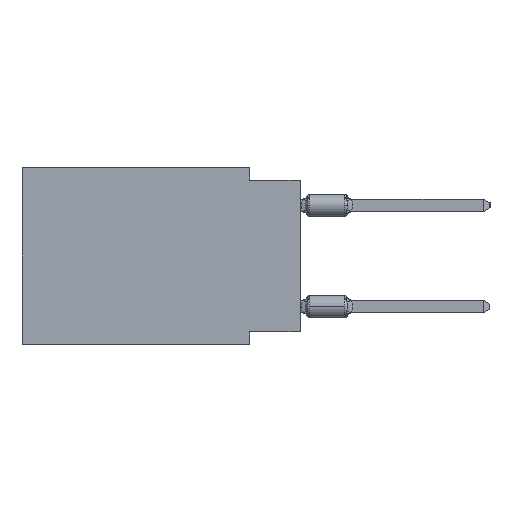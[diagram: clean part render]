
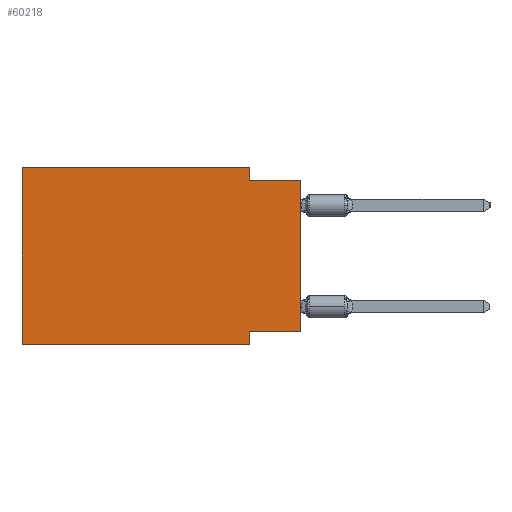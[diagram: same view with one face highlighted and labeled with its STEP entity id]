
A CAD part, left-side view. The second image highlights one B-rep face of the part: STEP entity #60218.
In plain terms, the highlighted planar face has unit normal (-1, 0, 0).
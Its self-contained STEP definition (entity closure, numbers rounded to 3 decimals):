
#1764 = CARTESIAN_POINT ( 'NONE',  ( 0., 0., -0.635 ) ) ;
#2218 = ORIENTED_EDGE ( 'NONE', *, *, #30671, .F. ) ;
#2288 = CARTESIAN_POINT ( 'NONE',  ( 0., 2.54, -8.89 ) ) ;
#2795 = ORIENTED_EDGE ( 'NONE', *, *, #37087, .T. ) ;
#5385 = DIRECTION ( 'NONE',  ( 0., 1., 0. ) ) ;
#5557 = VECTOR ( 'NONE', #57499, 1000. ) ;
#5923 = CARTESIAN_POINT ( 'NONE',  ( 0., 13.97, 0. ) ) ;
#6159 = CARTESIAN_POINT ( 'NONE',  ( 0., 13.97, -8.89 ) ) ;
#7140 = VERTEX_POINT ( 'NONE', #58990 ) ;
#9269 = PLANE ( 'NONE',  #31322 ) ;
#9578 = DIRECTION ( 'NONE',  ( 1., 0., 0. ) ) ;
#13674 = EDGE_CURVE ( 'NONE', #46646, #24754, #45529, .T. ) ;
#14096 = CARTESIAN_POINT ( 'NONE',  ( 0., 2.54, -8.89 ) ) ;
#14541 = ORIENTED_EDGE ( 'NONE', *, *, #25486, .T. ) ;
#15211 = ORIENTED_EDGE ( 'NONE', *, *, #61394, .F. ) ;
#15322 = VERTEX_POINT ( 'NONE', #14096 ) ;
#15597 = ORIENTED_EDGE ( 'NONE', *, *, #13674, .F. ) ;
#15773 = DIRECTION ( 'NONE',  ( 0., 0., 1. ) ) ;
#16227 = CARTESIAN_POINT ( 'NONE',  ( 0., 0., -8.255 ) ) ;
#18901 = CARTESIAN_POINT ( 'NONE',  ( 0., 13.97, 0. ) ) ;
#20080 = CARTESIAN_POINT ( 'NONE',  ( 0., 13.97, 0. ) ) ;
#21241 = DIRECTION ( 'NONE',  ( 0., 0., -1. ) ) ;
#22351 = CARTESIAN_POINT ( 'NONE',  ( 0., 0., -0.635 ) ) ;
#24740 = ORIENTED_EDGE ( 'NONE', *, *, #30100, .F. ) ;
#24754 = VERTEX_POINT ( 'NONE', #41744 ) ;
#24932 = ORIENTED_EDGE ( 'NONE', *, *, #27989, .F. ) ;
#25095 = VERTEX_POINT ( 'NONE', #38627 ) ;
#25486 = EDGE_CURVE ( 'NONE', #7140, #15322, #48722, .T. ) ;
#27989 = EDGE_CURVE ( 'NONE', #52520, #46646, #52221, .T. ) ;
#29491 = ORIENTED_EDGE ( 'NONE', *, *, #39081, .F. ) ;
#29633 = LINE ( 'NONE', #2288, #57215 ) ;
#30100 = EDGE_CURVE ( 'NONE', #7140, #52520, #43373, .T. ) ;
#30504 = VECTOR ( 'NONE', #34737, 1000. ) ;
#30671 = EDGE_CURVE ( 'NONE', #25095, #15322, #29633, .T. ) ;
#31322 = AXIS2_PLACEMENT_3D ( 'NONE', #18901, #9578, #40415 ) ;
#34737 = DIRECTION ( 'NONE',  ( 0., -1., 0. ) ) ;
#36470 = VECTOR ( 'NONE', #15773, 1000. ) ;
#36815 = DIRECTION ( 'NONE',  ( 0., 0., -1. ) ) ;
#37087 = EDGE_CURVE ( 'NONE', #42439, #51017, #59231, .T. ) ;
#38627 = CARTESIAN_POINT ( 'NONE',  ( 0., 2.54, -8.255 ) ) ;
#38903 = CARTESIAN_POINT ( 'NONE',  ( 0., 2.54, 0. ) ) ;
#39081 = EDGE_CURVE ( 'NONE', #42439, #25095, #42354, .T. ) ;
#39440 = VECTOR ( 'NONE', #48341, 1000. ) ;
#40415 = DIRECTION ( 'NONE',  ( 0., 0., -1. ) ) ;
#41550 = CARTESIAN_POINT ( 'NONE',  ( 0., 13.97, 0. ) ) ;
#41744 = CARTESIAN_POINT ( 'NONE',  ( 0., 2.54, -0.635 ) ) ;
#42354 = LINE ( 'NONE', #56957, #54360 ) ;
#42439 = VERTEX_POINT ( 'NONE', #16227 ) ;
#43373 = LINE ( 'NONE', #20080, #39440 ) ;
#44039 = CARTESIAN_POINT ( 'NONE',  ( 0., 0., 0. ) ) ;
#44750 = LINE ( 'NONE', #22351, #48274 ) ;
#45529 = LINE ( 'NONE', #60423, #47590 ) ;
#46646 = VERTEX_POINT ( 'NONE', #38903 ) ;
#46859 = FACE_OUTER_BOUND ( 'NONE', #58295, .T. ) ;
#47590 = VECTOR ( 'NONE', #36815, 1000. ) ;
#48274 = VECTOR ( 'NONE', #49401, 1000. ) ;
#48341 = DIRECTION ( 'NONE',  ( 0., 0., 1. ) ) ;
#48722 = LINE ( 'NONE', #6159, #30504 ) ;
#49401 = DIRECTION ( 'NONE',  ( 0., -1., 0. ) ) ;
#51017 = VERTEX_POINT ( 'NONE', #1764 ) ;
#52221 = LINE ( 'NONE', #5923, #5557 ) ;
#52520 = VERTEX_POINT ( 'NONE', #41550 ) ;
#54360 = VECTOR ( 'NONE', #5385, 1000. ) ;
#56957 = CARTESIAN_POINT ( 'NONE',  ( 0., 0., -8.255 ) ) ;
#57215 = VECTOR ( 'NONE', #21241, 1000. ) ;
#57499 = DIRECTION ( 'NONE',  ( 0., -1., 0. ) ) ;
#58295 = EDGE_LOOP ( 'NONE', ( #2795, #15211, #15597, #24932, #24740, #14541, #2218, #29491 ) ) ;
#58990 = CARTESIAN_POINT ( 'NONE',  ( 0., 13.97, -8.89 ) ) ;
#59231 = LINE ( 'NONE', #44039, #36470 ) ;
#60218 = ADVANCED_FACE ( 'NONE', ( #46859 ), #9269, .F. ) ;
#60423 = CARTESIAN_POINT ( 'NONE',  ( 0., 2.54, 0. ) ) ;
#61394 = EDGE_CURVE ( 'NONE', #24754, #51017, #44750, .T. ) ;
